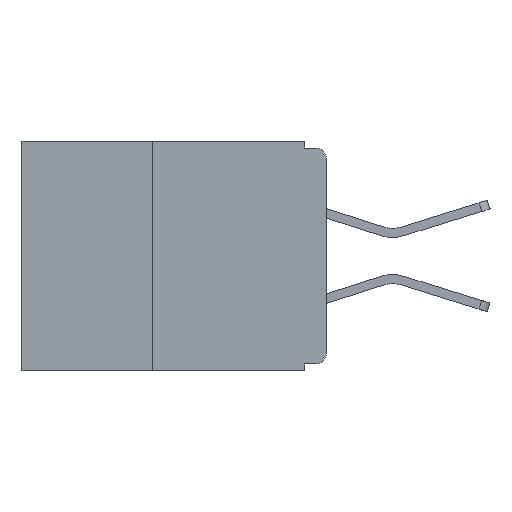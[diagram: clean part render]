
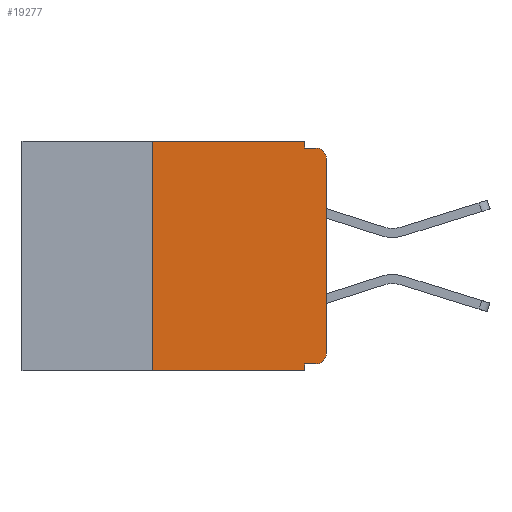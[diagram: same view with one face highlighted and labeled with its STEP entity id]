
A CAD part, left-side view. The second image highlights one B-rep face of the part: STEP entity #19277.
In plain terms, the highlighted planar face has unit normal (-1, 0, 0).
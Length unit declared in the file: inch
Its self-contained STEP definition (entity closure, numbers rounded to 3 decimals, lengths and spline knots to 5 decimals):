
#174 = LINE ( 'NONE', #29881, #21473 ) ;
#457 = CARTESIAN_POINT ( 'NONE',  ( 0., 0.25, -0.33 ) ) ;
#746 = CARTESIAN_POINT ( 'NONE',  ( 0., 0.015, -0.01 ) ) ;
#1447 = EDGE_CURVE ( 'NONE', #16520, #19991, #15382, .T. ) ;
#1842 = CARTESIAN_POINT ( 'NONE',  ( 0., 0.015, -0.305 ) ) ;
#1895 = VERTEX_POINT ( 'NONE', #11266 ) ;
#2422 = ORIENTED_EDGE ( 'NONE', *, *, #10419, .T. ) ;
#2570 = CARTESIAN_POINT ( 'NONE',  ( 0., 0.031, 0. ) ) ;
#3615 = ORIENTED_EDGE ( 'NONE', *, *, #7408, .F. ) ;
#3627 = LINE ( 'NONE', #27242, #29898 ) ;
#4378 = DIRECTION ( 'NONE',  ( 0., 0., -1. ) ) ;
#4597 = VECTOR ( 'NONE', #22815, 39.37008 ) ;
#4652 = DIRECTION ( 'NONE',  ( 0., 0., -1. ) ) ;
#4999 = CARTESIAN_POINT ( 'NONE',  ( 0., 0., 0. ) ) ;
#5011 = VECTOR ( 'NONE', #29582, 39.37008 ) ;
#5379 = CARTESIAN_POINT ( 'NONE',  ( 0., 0.031, -0.33 ) ) ;
#5431 = EDGE_CURVE ( 'NONE', #14500, #1895, #10054, .T. ) ;
#6013 = CARTESIAN_POINT ( 'NONE',  ( 0., 0.25, -0.33 ) ) ;
#6342 = EDGE_CURVE ( 'NONE', #24329, #24445, #8471, .T. ) ;
#6650 = DIRECTION ( 'NONE',  ( 1., 0., 0. ) ) ;
#6751 = ORIENTED_EDGE ( 'NONE', *, *, #29713, .F. ) ;
#7153 = DIRECTION ( 'NONE',  ( -1., 0., 0. ) ) ;
#7325 = FACE_OUTER_BOUND ( 'NONE', #29862, .T. ) ;
#7408 = EDGE_CURVE ( 'NONE', #24329, #14500, #11090, .T. ) ;
#8015 = VERTEX_POINT ( 'NONE', #746 ) ;
#8384 = CARTESIAN_POINT ( 'NONE',  ( 0., 0.031, -0.32 ) ) ;
#8457 = EDGE_CURVE ( 'NONE', #24445, #11983, #18096, .T. ) ;
#8471 = CIRCLE ( 'NONE', #16785, 0.015 ) ;
#8523 = DIRECTION ( 'NONE',  ( 0., 0., 1. ) ) ;
#10030 = DIRECTION ( 'NONE',  ( 0., -1., 0. ) ) ;
#10054 = LINE ( 'NONE', #5379, #22392 ) ;
#10419 = EDGE_CURVE ( 'NONE', #14018, #1895, #174, .T. ) ;
#11090 = LINE ( 'NONE', #25455, #29955 ) ;
#11266 = CARTESIAN_POINT ( 'NONE',  ( 0., 0.031, -0.33 ) ) ;
#11983 = VERTEX_POINT ( 'NONE', #14024 ) ;
#12513 = ORIENTED_EDGE ( 'NONE', *, *, #1447, .F. ) ;
#13274 = ORIENTED_EDGE ( 'NONE', *, *, #6342, .T. ) ;
#14018 = VERTEX_POINT ( 'NONE', #457 ) ;
#14024 = CARTESIAN_POINT ( 'NONE',  ( 0., 0., -0.025 ) ) ;
#14350 = DIRECTION ( 'NONE',  ( 0., 0., -1. ) ) ;
#14500 = VERTEX_POINT ( 'NONE', #8384 ) ;
#14755 = CARTESIAN_POINT ( 'NONE',  ( 0., 0.25, 0. ) ) ;
#14912 = VERTEX_POINT ( 'NONE', #14755 ) ;
#15382 = LINE ( 'NONE', #2570, #28515 ) ;
#16259 = CARTESIAN_POINT ( 'NONE',  ( 0., 0.031, 0. ) ) ;
#16520 = VERTEX_POINT ( 'NONE', #16259 ) ;
#16785 = AXIS2_PLACEMENT_3D ( 'NONE', #1842, #19116, #4378 ) ;
#17565 = DIRECTION ( 'NONE',  ( 0., -1., 0. ) ) ;
#17605 = LINE ( 'NONE', #6013, #23434 ) ;
#18002 = AXIS2_PLACEMENT_3D ( 'NONE', #21385, #6650, #23879 ) ;
#18096 = LINE ( 'NONE', #4999, #5011 ) ;
#19116 = DIRECTION ( 'NONE',  ( -1., 0., 0. ) ) ;
#19277 = ADVANCED_FACE ( 'NONE', ( #7325 ), #26241, .F. ) ;
#19389 = CARTESIAN_POINT ( 'NONE',  ( 0., 0.015, -0.32 ) ) ;
#19991 = VERTEX_POINT ( 'NONE', #24305 ) ;
#20288 = CARTESIAN_POINT ( 'NONE',  ( 0., 0., -0.01 ) ) ;
#20924 = AXIS2_PLACEMENT_3D ( 'NONE', #21878, #7153, #24353 ) ;
#20970 = ORIENTED_EDGE ( 'NONE', *, *, #5431, .F. ) ;
#21183 = EDGE_CURVE ( 'NONE', #11983, #8015, #28329, .T. ) ;
#21385 = CARTESIAN_POINT ( 'NONE',  ( 0., 0.437, 0. ) ) ;
#21473 = VECTOR ( 'NONE', #17565, 39.37008 ) ;
#21878 = CARTESIAN_POINT ( 'NONE',  ( 0., 0.015, -0.025 ) ) ;
#22392 = VECTOR ( 'NONE', #4652, 39.37008 ) ;
#22463 = CARTESIAN_POINT ( 'NONE',  ( 0., 0., -0.305 ) ) ;
#22815 = DIRECTION ( 'NONE',  ( 0., -1., 0. ) ) ;
#23312 = ORIENTED_EDGE ( 'NONE', *, *, #23902, .F. ) ;
#23434 = VECTOR ( 'NONE', #8523, 39.37008 ) ;
#23879 = DIRECTION ( 'NONE',  ( 0., 0., -1. ) ) ;
#23902 = EDGE_CURVE ( 'NONE', #19991, #8015, #30808, .T. ) ;
#24305 = CARTESIAN_POINT ( 'NONE',  ( 0., 0.031, -0.01 ) ) ;
#24329 = VERTEX_POINT ( 'NONE', #19389 ) ;
#24353 = DIRECTION ( 'NONE',  ( 0., 0., -1. ) ) ;
#24445 = VERTEX_POINT ( 'NONE', #22463 ) ;
#25274 = EDGE_CURVE ( 'NONE', #14018, #14912, #17605, .T. ) ;
#25455 = CARTESIAN_POINT ( 'NONE',  ( 0., 0., -0.32 ) ) ;
#26241 = PLANE ( 'NONE',  #18002 ) ;
#26384 = ORIENTED_EDGE ( 'NONE', *, *, #25274, .F. ) ;
#26755 = ORIENTED_EDGE ( 'NONE', *, *, #21183, .T. ) ;
#27242 = CARTESIAN_POINT ( 'NONE',  ( 0., 0.437, 0. ) ) ;
#27926 = DIRECTION ( 'NONE',  ( 0., 1., 0. ) ) ;
#28329 = CIRCLE ( 'NONE', #20924, 0.015 ) ;
#28515 = VECTOR ( 'NONE', #14350, 39.37008 ) ;
#29582 = DIRECTION ( 'NONE',  ( 0., 0., 1. ) ) ;
#29713 = EDGE_CURVE ( 'NONE', #14912, #16520, #3627, .T. ) ;
#29862 = EDGE_LOOP ( 'NONE', ( #30960, #26755, #23312, #12513, #6751, #26384, #2422, #20970, #3615, #13274 ) ) ;
#29881 = CARTESIAN_POINT ( 'NONE',  ( 0., 0.437, -0.33 ) ) ;
#29898 = VECTOR ( 'NONE', #10030, 39.37008 ) ;
#29955 = VECTOR ( 'NONE', #27926, 39.37008 ) ;
#30808 = LINE ( 'NONE', #20288, #4597 ) ;
#30960 = ORIENTED_EDGE ( 'NONE', *, *, #8457, .T. ) ;
